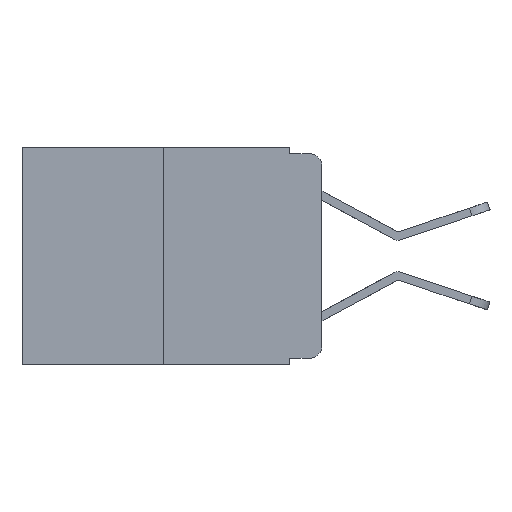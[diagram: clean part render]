
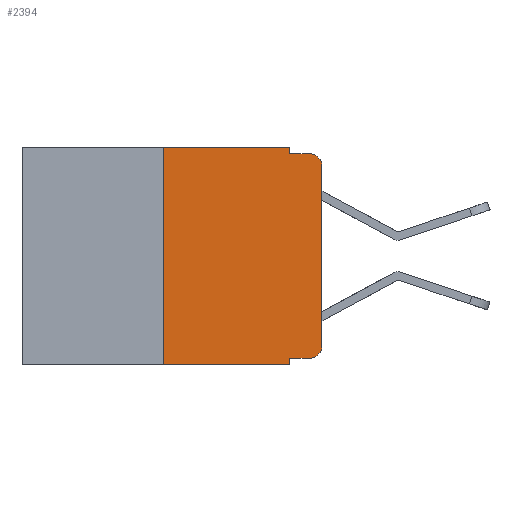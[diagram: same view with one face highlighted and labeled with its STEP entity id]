
A CAD part, left-side view. The second image highlights one B-rep face of the part: STEP entity #2394.
In plain terms, the highlighted planar face has unit normal (-1, 0, 0).
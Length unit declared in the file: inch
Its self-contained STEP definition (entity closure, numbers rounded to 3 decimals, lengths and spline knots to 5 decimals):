
#606 = DIRECTION ( 'NONE',  ( 0., 0., -1. ) ) ;
#729 = EDGE_CURVE ( 'NONE', #1790, #4823, #11634, .T. ) ;
#745 = DIRECTION ( 'NONE',  ( 0., 0., -1. ) ) ;
#758 = ORIENTED_EDGE ( 'NONE', *, *, #8875, .T. ) ;
#760 = DIRECTION ( 'NONE',  ( 0., -1., 0. ) ) ;
#792 = DIRECTION ( 'NONE',  ( 1., 0., 0. ) ) ;
#1098 = CARTESIAN_POINT ( 'NONE',  ( 0., 0.473, 0. ) ) ;
#1189 = CARTESIAN_POINT ( 'NONE',  ( 0., 0.25, 0. ) ) ;
#1263 = PLANE ( 'NONE',  #5615 ) ;
#1561 = LINE ( 'NONE', #5777, #6215 ) ;
#1641 = EDGE_LOOP ( 'NONE', ( #6832, #9333, #1909, #12168, #9940, #2568, #3176, #5787, #8309, #758 ) ) ;
#1790 = VERTEX_POINT ( 'NONE', #9650 ) ;
#1909 = ORIENTED_EDGE ( 'NONE', *, *, #12701, .F. ) ;
#1937 = VECTOR ( 'NONE', #10930, 39.37008 ) ;
#2058 = CARTESIAN_POINT ( 'NONE',  ( 0., 0.051, 0. ) ) ;
#2130 = EDGE_CURVE ( 'NONE', #4869, #1790, #10456, .T. ) ;
#2265 = CARTESIAN_POINT ( 'NONE',  ( 0., 0.051, -0.01 ) ) ;
#2327 = CARTESIAN_POINT ( 'NONE',  ( 0., 0.25, 0. ) ) ;
#2394 = ADVANCED_FACE ( 'NONE', ( #7455 ), #1263, .F. ) ;
#2568 = ORIENTED_EDGE ( 'NONE', *, *, #10804, .F. ) ;
#2630 = LINE ( 'NONE', #12371, #4908 ) ;
#2918 = CARTESIAN_POINT ( 'NONE',  ( 0., 0.051, -0.343 ) ) ;
#2942 = CIRCLE ( 'NONE', #7991, 0.02 ) ;
#3051 = DIRECTION ( 'NONE',  ( 0., 0., -1. ) ) ;
#3176 = ORIENTED_EDGE ( 'NONE', *, *, #4550, .T. ) ;
#3948 = VERTEX_POINT ( 'NONE', #9422 ) ;
#4476 = VECTOR ( 'NONE', #760, 39.37008 ) ;
#4550 = EDGE_CURVE ( 'NONE', #7124, #4871, #5567, .T. ) ;
#4823 = VERTEX_POINT ( 'NONE', #11100 ) ;
#4869 = VERTEX_POINT ( 'NONE', #10705 ) ;
#4871 = VERTEX_POINT ( 'NONE', #2918 ) ;
#4884 = LINE ( 'NONE', #1189, #1937 ) ;
#4908 = VECTOR ( 'NONE', #6686, 39.37008 ) ;
#5567 = LINE ( 'NONE', #9212, #8109 ) ;
#5615 = AXIS2_PLACEMENT_3D ( 'NONE', #1098, #792, #745 ) ;
#5774 = CARTESIAN_POINT ( 'NONE',  ( 0., 0.051, -0.333 ) ) ;
#5777 = CARTESIAN_POINT ( 'NONE',  ( 0., 0.051, 0. ) ) ;
#5787 = ORIENTED_EDGE ( 'NONE', *, *, #10160, .F. ) ;
#6034 = VECTOR ( 'NONE', #11746, 39.37008 ) ;
#6215 = VECTOR ( 'NONE', #11467, 39.37008 ) ;
#6609 = DIRECTION ( 'NONE',  ( -1., 0., 0. ) ) ;
#6686 = DIRECTION ( 'NONE',  ( 0., 0., -1. ) ) ;
#6769 = EDGE_CURVE ( 'NONE', #10864, #11512, #9435, .T. ) ;
#6811 = DIRECTION ( 'NONE',  ( -1., 0., 0. ) ) ;
#6832 = ORIENTED_EDGE ( 'NONE', *, *, #2130, .T. ) ;
#7122 = DIRECTION ( 'NONE',  ( 0., -1., 0. ) ) ;
#7124 = VERTEX_POINT ( 'NONE', #9327 ) ;
#7387 = LINE ( 'NONE', #8094, #9601 ) ;
#7455 = FACE_OUTER_BOUND ( 'NONE', #1641, .T. ) ;
#7691 = AXIS2_PLACEMENT_3D ( 'NONE', #7919, #6811, #3051 ) ;
#7851 = DIRECTION ( 'NONE',  ( 0., 0., 1. ) ) ;
#7919 = CARTESIAN_POINT ( 'NONE',  ( 0., 0.02, -0.03 ) ) ;
#7991 = AXIS2_PLACEMENT_3D ( 'NONE', #12288, #6609, #606 ) ;
#8094 = CARTESIAN_POINT ( 'NONE',  ( 0., 0.051, -0.01 ) ) ;
#8109 = VECTOR ( 'NONE', #8457, 39.37008 ) ;
#8200 = VECTOR ( 'NONE', #7851, 39.37008 ) ;
#8208 = LINE ( 'NONE', #5774, #4476 ) ;
#8309 = ORIENTED_EDGE ( 'NONE', *, *, #9506, .T. ) ;
#8453 = CARTESIAN_POINT ( 'NONE',  ( 0., 0., 0. ) ) ;
#8457 = DIRECTION ( 'NONE',  ( 0., -1., 0. ) ) ;
#8833 = CARTESIAN_POINT ( 'NONE',  ( 0., 0.02, -0.333 ) ) ;
#8875 = EDGE_CURVE ( 'NONE', #12591, #4869, #2942, .T. ) ;
#9212 = CARTESIAN_POINT ( 'NONE',  ( 0., 0.473, -0.343 ) ) ;
#9327 = CARTESIAN_POINT ( 'NONE',  ( 0., 0.25, -0.343 ) ) ;
#9333 = ORIENTED_EDGE ( 'NONE', *, *, #729, .T. ) ;
#9422 = CARTESIAN_POINT ( 'NONE',  ( 0., 0.051, -0.333 ) ) ;
#9435 = LINE ( 'NONE', #10811, #6034 ) ;
#9506 = EDGE_CURVE ( 'NONE', #3948, #12591, #8208, .T. ) ;
#9601 = VECTOR ( 'NONE', #7122, 39.37008 ) ;
#9650 = CARTESIAN_POINT ( 'NONE',  ( 0., 0., -0.03 ) ) ;
#9707 = VERTEX_POINT ( 'NONE', #2265 ) ;
#9940 = ORIENTED_EDGE ( 'NONE', *, *, #6769, .F. ) ;
#10160 = EDGE_CURVE ( 'NONE', #3948, #4871, #2630, .T. ) ;
#10456 = LINE ( 'NONE', #8453, #8200 ) ;
#10705 = CARTESIAN_POINT ( 'NONE',  ( 0., 0., -0.313 ) ) ;
#10804 = EDGE_CURVE ( 'NONE', #7124, #10864, #4884, .T. ) ;
#10811 = CARTESIAN_POINT ( 'NONE',  ( 0., 0.473, 0. ) ) ;
#10864 = VERTEX_POINT ( 'NONE', #2327 ) ;
#10930 = DIRECTION ( 'NONE',  ( 0., 0., 1. ) ) ;
#11100 = CARTESIAN_POINT ( 'NONE',  ( 0., 0.02, -0.01 ) ) ;
#11467 = DIRECTION ( 'NONE',  ( 0., 0., -1. ) ) ;
#11512 = VERTEX_POINT ( 'NONE', #2058 ) ;
#11634 = CIRCLE ( 'NONE', #7691, 0.02 ) ;
#11746 = DIRECTION ( 'NONE',  ( 0., -1., 0. ) ) ;
#12052 = EDGE_CURVE ( 'NONE', #11512, #9707, #1561, .T. ) ;
#12168 = ORIENTED_EDGE ( 'NONE', *, *, #12052, .F. ) ;
#12288 = CARTESIAN_POINT ( 'NONE',  ( 0., 0.02, -0.313 ) ) ;
#12371 = CARTESIAN_POINT ( 'NONE',  ( 0., 0.051, 0. ) ) ;
#12591 = VERTEX_POINT ( 'NONE', #8833 ) ;
#12701 = EDGE_CURVE ( 'NONE', #9707, #4823, #7387, .T. ) ;
